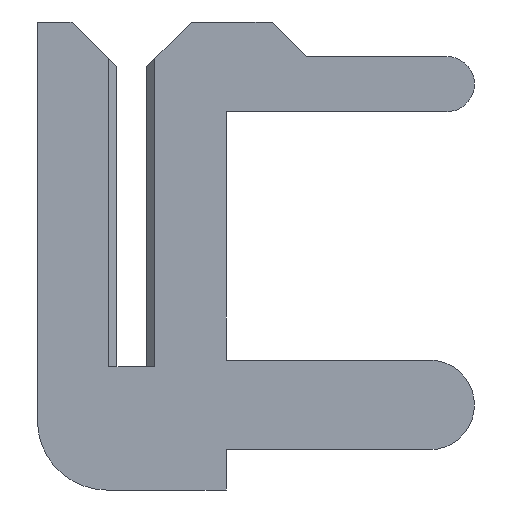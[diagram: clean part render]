
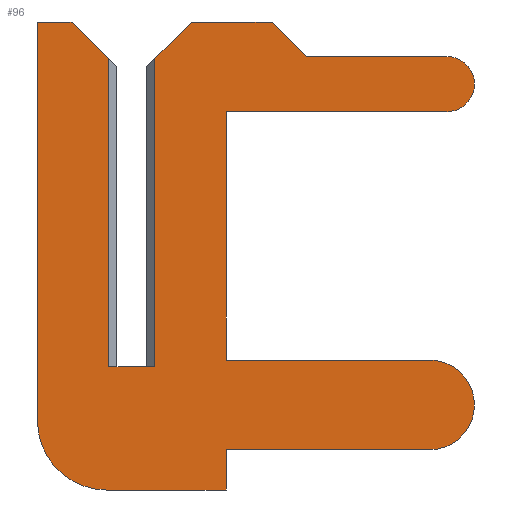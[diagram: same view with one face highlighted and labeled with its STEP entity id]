
A CAD part, left-side view. The second image highlights one B-rep face of the part: STEP entity #96.
In plain terms, the highlighted planar face has unit normal (-1, 0, 0).
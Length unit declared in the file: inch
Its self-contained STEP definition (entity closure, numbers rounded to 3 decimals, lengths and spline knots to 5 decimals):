
#16 = LINE ( 'NONE', #378, #523 ) ;
#17 = CARTESIAN_POINT ( 'NONE',  ( -0.01, 0.0065, 0.1305 ) ) ;
#21 = EDGE_CURVE ( 'NONE', #1275, #970, #590, .T. ) ;
#44 = VERTEX_POINT ( 'NONE', #680 ) ;
#51 = LINE ( 'NONE', #816, #1183 ) ;
#54 = CARTESIAN_POINT ( 'NONE',  ( -0.01, 0.026, 0.15 ) ) ;
#73 = EDGE_CURVE ( 'NONE', #864, #164, #775, .T. ) ;
#77 = DIRECTION ( 'NONE',  ( 0., 0., -1. ) ) ;
#96 = ADVANCED_FACE ( 'NONE', ( #454 ), #1271, .T. ) ;
#115 = ORIENTED_EDGE ( 'NONE', *, *, #288, .F. ) ;
#122 = AXIS2_PLACEMENT_3D ( 'NONE', #276, #986, #1090 ) ;
#125 = ORIENTED_EDGE ( 'NONE', *, *, #547, .F. ) ;
#131 = DIRECTION ( 'NONE',  ( 0., 0., 1. ) ) ;
#137 = ORIENTED_EDGE ( 'NONE', *, *, #1091, .F. ) ;
#139 = DIRECTION ( 'NONE',  ( 1., 0., 0. ) ) ;
#157 = ORIENTED_EDGE ( 'NONE', *, *, #960, .F. ) ;
#163 = LINE ( 'NONE', #1448, #1224 ) ;
#164 = VERTEX_POINT ( 'NONE', #1180 ) ;
#168 = CARTESIAN_POINT ( 'NONE',  ( -0.01, 0.026, 0.15 ) ) ;
#189 = VERTEX_POINT ( 'NONE', #254 ) ;
#201 = ORIENTED_EDGE ( 'NONE', *, *, #725, .F. ) ;
#213 = EDGE_CURVE ( 'NONE', #869, #1047, #16, .T. ) ;
#222 = VECTOR ( 'NONE', #249, 39.37008 ) ;
#227 = VECTOR ( 'NONE', #77, 39.37008 ) ;
#229 = EDGE_CURVE ( 'NONE', #1201, #895, #734, .T. ) ;
#237 = VECTOR ( 'NONE', #1408, 39.37008 ) ;
#242 = DIRECTION ( 'NONE',  ( 0., -0.707, -0.707 ) ) ;
#245 = CARTESIAN_POINT ( 'NONE',  ( -0.01, -0.1295, -0.0165 ) ) ;
#249 = DIRECTION ( 'NONE',  ( 0., -1., 0. ) ) ;
#253 = VECTOR ( 'NONE', #1033, 39.37008 ) ;
#254 = CARTESIAN_POINT ( 'NONE',  ( -0.01, -0.026, 0.15 ) ) ;
#262 = EDGE_CURVE ( 'NONE', #1087, #970, #1110, .T. ) ;
#276 = CARTESIAN_POINT ( 'NONE',  ( -0.01, -0.137, 0.123 ) ) ;
#288 = EDGE_CURVE ( 'NONE', #189, #704, #1292, .T. ) ;
#293 = CARTESIAN_POINT ( 'NONE',  ( -0.01, 0.041, 0.15 ) ) ;
#298 = CARTESIAN_POINT ( 'NONE',  ( -0.01, -0.076, 0.135 ) ) ;
#302 = DIRECTION ( 'NONE',  ( 0., 1., 0. ) ) ;
#315 = EDGE_CURVE ( 'NONE', #1182, #44, #51, .T. ) ;
#320 = CARTESIAN_POINT ( 'NONE',  ( -0.01, -0.01, 0. ) ) ;
#366 = VECTOR ( 'NONE', #908, 39.37008 ) ;
#374 = CARTESIAN_POINT ( 'NONE',  ( -0.01, 0.011, -0.0235 ) ) ;
#378 = CARTESIAN_POINT ( 'NONE',  ( -0.01, -0.041, -0.0535 ) ) ;
#387 = CARTESIAN_POINT ( 'NONE',  ( -0.01, 0.01, -0.0235 ) ) ;
#397 = CARTESIAN_POINT ( 'NONE',  ( -0.01, -0.041, -0.036 ) ) ;
#399 = VECTOR ( 'NONE', #1060, 39.37008 ) ;
#402 = EDGE_CURVE ( 'NONE', #1311, #1097, #543, .T. ) ;
#423 = ORIENTED_EDGE ( 'NONE', *, *, #829, .F. ) ;
#435 = CARTESIAN_POINT ( 'NONE',  ( -0.01, -0.041, -0.0535 ) ) ;
#440 = CARTESIAN_POINT ( 'NONE',  ( -0.01, 0.01, 0. ) ) ;
#442 = ORIENTED_EDGE ( 'NONE', *, *, #806, .F. ) ;
#454 = FACE_OUTER_BOUND ( 'NONE', #1395, .T. ) ;
#474 = CARTESIAN_POINT ( 'NONE',  ( -0.01, 0.0065, 0. ) ) ;
#488 = CIRCLE ( 'NONE', #1109, 0.0195 ) ;
#495 = DIRECTION ( 'NONE',  ( 0., 0., -1. ) ) ;
#499 = ORIENTED_EDGE ( 'NONE', *, *, #402, .F. ) ;
#500 = VECTOR ( 'NONE', #763, 39.37008 ) ;
#523 = VECTOR ( 'NONE', #495, 39.37008 ) ;
#543 = LINE ( 'NONE', #1393, #1166 ) ;
#547 = EDGE_CURVE ( 'NONE', #1097, #842, #488, .T. ) ;
#556 = ORIENTED_EDGE ( 'NONE', *, *, #229, .F. ) ;
#565 = ORIENTED_EDGE ( 'NONE', *, *, #1234, .F. ) ;
#590 = LINE ( 'NONE', #793, #253 ) ;
#592 = ORIENTED_EDGE ( 'NONE', *, *, #1245, .F. ) ;
#599 = DIRECTION ( 'NONE',  ( -1., 0., 0. ) ) ;
#604 = CARTESIAN_POINT ( 'NONE',  ( -0.01, 0.011, -0.0535 ) ) ;
#624 = AXIS2_PLACEMENT_3D ( 'NONE', #374, #961, #1065 ) ;
#654 = CARTESIAN_POINT ( 'NONE',  ( -0.01, -0.041, 0.003 ) ) ;
#658 = CARTESIAN_POINT ( 'NONE',  ( -0.01, 0.041, -0.0235 ) ) ;
#661 = VECTOR ( 'NONE', #242, 39.37008 ) ;
#666 = DIRECTION ( 'NONE',  ( 0., -0.707, -0.707 ) ) ;
#680 = CARTESIAN_POINT ( 'NONE',  ( -0.01, -0.137, 0.135 ) ) ;
#704 = VERTEX_POINT ( 'NONE', #1411 ) ;
#725 = EDGE_CURVE ( 'NONE', #1077, #1118, #1017, .T. ) ;
#732 = ORIENTED_EDGE ( 'NONE', *, *, #73, .F. ) ;
#734 = LINE ( 'NONE', #944, #399 ) ;
#741 = ORIENTED_EDGE ( 'NONE', *, *, #213, .F. ) ;
#755 = EDGE_CURVE ( 'NONE', #1087, #164, #760, .T. ) ;
#760 = LINE ( 'NONE', #387, #1262 ) ;
#763 = DIRECTION ( 'NONE',  ( 0., -0.707, 0.707 ) ) ;
#775 = LINE ( 'NONE', #17, #661 ) ;
#793 = CARTESIAN_POINT ( 'NONE',  ( -0.01, -0.01, 0.15 ) ) ;
#806 = EDGE_CURVE ( 'NONE', #1047, #1077, #1394, .T. ) ;
#816 = CARTESIAN_POINT ( 'NONE',  ( -0.01, -0.137, 0.135 ) ) ;
#829 = EDGE_CURVE ( 'NONE', #1118, #1229, #163, .T. ) ;
#830 = DIRECTION ( 'NONE',  ( 0., 0., 1. ) ) ;
#833 = DIRECTION ( 'NONE',  ( 0., -1., 0. ) ) ;
#835 = LINE ( 'NONE', #397, #1425 ) ;
#842 = VERTEX_POINT ( 'NONE', #995 ) ;
#843 = LINE ( 'NONE', #654, #227 ) ;
#846 = DIRECTION ( 'NONE',  ( 0., 1., 0. ) ) ;
#859 = EDGE_CURVE ( 'NONE', #44, #1201, #1416, .T. ) ;
#864 = VERTEX_POINT ( 'NONE', #54 ) ;
#867 = CARTESIAN_POINT ( 'NONE',  ( -0.01, -0.041, -0.036 ) ) ;
#869 = VERTEX_POINT ( 'NONE', #867 ) ;
#889 = EDGE_CURVE ( 'NONE', #842, #869, #835, .T. ) ;
#895 = VERTEX_POINT ( 'NONE', #1427 ) ;
#908 = DIRECTION ( 'NONE',  ( 0., -1., 0. ) ) ;
#930 = CARTESIAN_POINT ( 'NONE',  ( -0.01, -0.137, 0.111 ) ) ;
#944 = CARTESIAN_POINT ( 'NONE',  ( -0.01, -0.041, 0.111 ) ) ;
#952 = DIRECTION ( 'NONE',  ( 0., 0., 1. ) ) ;
#960 = EDGE_CURVE ( 'NONE', #1229, #864, #1337, .T. ) ;
#961 = DIRECTION ( 'NONE',  ( 1., 0., 0. ) ) ;
#968 = ORIENTED_EDGE ( 'NONE', *, *, #315, .F. ) ;
#970 = VERTEX_POINT ( 'NONE', #320 ) ;
#986 = DIRECTION ( 'NONE',  ( 1., 0., 0. ) ) ;
#995 = CARTESIAN_POINT ( 'NONE',  ( -0.01, -0.1295, -0.036 ) ) ;
#1004 = AXIS2_PLACEMENT_3D ( 'NONE', #1172, #599, #131 ) ;
#1016 = CARTESIAN_POINT ( 'NONE',  ( -0.01, -0.1295, 0.003 ) ) ;
#1017 = CIRCLE ( 'NONE', #624, 0.03 ) ;
#1024 = LINE ( 'NONE', #298, #1231 ) ;
#1033 = DIRECTION ( 'NONE',  ( 0., 0., -1. ) ) ;
#1047 = VERTEX_POINT ( 'NONE', #435 ) ;
#1055 = ORIENTED_EDGE ( 'NONE', *, *, #262, .F. ) ;
#1060 = DIRECTION ( 'NONE',  ( 0., 1., 0. ) ) ;
#1065 = DIRECTION ( 'NONE',  ( 0., 0., 1. ) ) ;
#1068 = CARTESIAN_POINT ( 'NONE',  ( -0.01, -0.026, 0.15 ) ) ;
#1076 = DIRECTION ( 'NONE',  ( 0., -1., 0. ) ) ;
#1077 = VERTEX_POINT ( 'NONE', #1133 ) ;
#1079 = CARTESIAN_POINT ( 'NONE',  ( -0.01, -0.041, 0.003 ) ) ;
#1087 = VERTEX_POINT ( 'NONE', #440 ) ;
#1090 = DIRECTION ( 'NONE',  ( 0., 0., 1. ) ) ;
#1091 = EDGE_CURVE ( 'NONE', #1275, #189, #1158, .T. ) ;
#1092 = CARTESIAN_POINT ( 'NONE',  ( -0.01, -0.076, 0.135 ) ) ;
#1097 = VERTEX_POINT ( 'NONE', #1016 ) ;
#1109 = AXIS2_PLACEMENT_3D ( 'NONE', #245, #139, #830 ) ;
#1110 = LINE ( 'NONE', #474, #222 ) ;
#1114 = DIRECTION ( 'NONE',  ( 0., 0., 1. ) ) ;
#1118 = VERTEX_POINT ( 'NONE', #658 ) ;
#1126 = CARTESIAN_POINT ( 'NONE',  ( -0.01, -0.0065, 0.1305 ) ) ;
#1133 = CARTESIAN_POINT ( 'NONE',  ( -0.01, 0.011, -0.0535 ) ) ;
#1158 = LINE ( 'NONE', #1126, #500 ) ;
#1166 = VECTOR ( 'NONE', #1076, 39.37008 ) ;
#1172 = CARTESIAN_POINT ( 'NONE',  ( -0.01, 0.011, -0.0235 ) ) ;
#1180 = CARTESIAN_POINT ( 'NONE',  ( -0.01, 0.01, 0.134 ) ) ;
#1182 = VERTEX_POINT ( 'NONE', #1092 ) ;
#1183 = VECTOR ( 'NONE', #833, 39.37008 ) ;
#1201 = VERTEX_POINT ( 'NONE', #930 ) ;
#1202 = ORIENTED_EDGE ( 'NONE', *, *, #755, .T. ) ;
#1205 = ORIENTED_EDGE ( 'NONE', *, *, #859, .F. ) ;
#1210 = ORIENTED_EDGE ( 'NONE', *, *, #21, .T. ) ;
#1224 = VECTOR ( 'NONE', #1114, 39.37008 ) ;
#1229 = VERTEX_POINT ( 'NONE', #293 ) ;
#1231 = VECTOR ( 'NONE', #666, 39.37008 ) ;
#1234 = EDGE_CURVE ( 'NONE', #704, #1182, #1024, .T. ) ;
#1238 = ORIENTED_EDGE ( 'NONE', *, *, #889, .F. ) ;
#1245 = EDGE_CURVE ( 'NONE', #895, #1311, #843, .T. ) ;
#1262 = VECTOR ( 'NONE', #952, 39.37008 ) ;
#1271 = PLANE ( 'NONE',  #1004 ) ;
#1275 = VERTEX_POINT ( 'NONE', #1281 ) ;
#1281 = CARTESIAN_POINT ( 'NONE',  ( -0.01, -0.01, 0.134 ) ) ;
#1292 = LINE ( 'NONE', #1068, #237 ) ;
#1311 = VERTEX_POINT ( 'NONE', #1079 ) ;
#1337 = LINE ( 'NONE', #168, #366 ) ;
#1380 = VECTOR ( 'NONE', #846, 39.37008 ) ;
#1393 = CARTESIAN_POINT ( 'NONE',  ( -0.01, -0.1295, 0.003 ) ) ;
#1394 = LINE ( 'NONE', #604, #1380 ) ;
#1395 = EDGE_LOOP ( 'NONE', ( #137, #1210, #1055, #1202, #732, #157, #423, #201, #442, #741, #1238, #125, #499, #592, #556, #1205, #968, #565, #115 ) ) ;
#1408 = DIRECTION ( 'NONE',  ( 0., -1., 0. ) ) ;
#1411 = CARTESIAN_POINT ( 'NONE',  ( -0.01, -0.061, 0.15 ) ) ;
#1416 = CIRCLE ( 'NONE', #122, 0.012 ) ;
#1425 = VECTOR ( 'NONE', #302, 39.37008 ) ;
#1427 = CARTESIAN_POINT ( 'NONE',  ( -0.01, -0.041, 0.111 ) ) ;
#1448 = CARTESIAN_POINT ( 'NONE',  ( -0.01, 0.041, 0.15 ) ) ;
